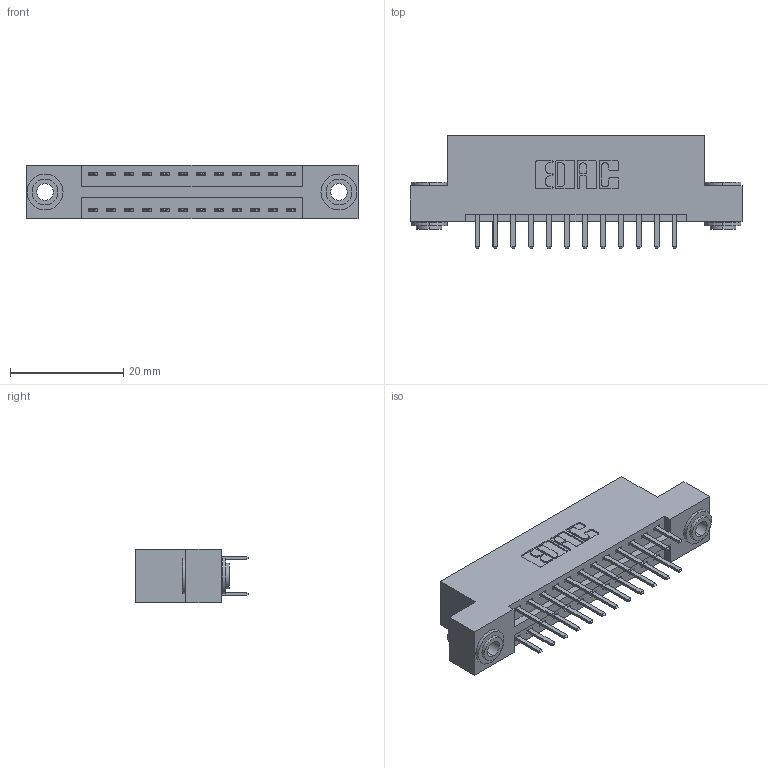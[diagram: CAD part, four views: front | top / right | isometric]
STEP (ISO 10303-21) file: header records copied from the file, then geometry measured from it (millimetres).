
FILE_DESCRIPTION (( 'STEP AP203' ), '1' );
FILE_NAME ('346-024-520-203.STEP', '2022-05-18T22:43:21', ( '' ), ( '' ), 'SwSTEP 2.0', 'SolidWorks 2020', '' );
FILE_SCHEMA (( 'CONFIG_CONTROL_DESIGN' ));
Length unit declared in the file: inch
Products named in the file (4): 345-292-001_345-293-120; 345-250-002_345-250-002-102; 346 Part_Flush Mounting Lugs - 0.156 Dia-TH; 346-024-520-203
Assembly tree (27 placements, depth 2):
  346-024-520-203
    346 Part_Flush Mounting Lugs - 0.156 Dia-TH
    345-292-001_345-293-120  x24
    345-250-002_345-250-002-102  x2
Bounding box: 58.67 x 20.02 x 9.4 mm (x, y, z)
Volume: 5479.2 mm3; surface area: 7284 mm2
Topology: 27 solids, 27 shells, 1518 faces, 4353 edges, 2834 vertices
Faces by surface type: plane 988, cylinder 522, cone 8
Entity records: 13050 total; most frequent: CARTESIAN_POINT 2185, ORIENTED_EDGE 2098, DIRECTION 1995, EDGE_CURVE 1049, LINE 841, VECTOR 841, VERTEX_POINT 694, AXIS2_PLACEMENT_3D 577
